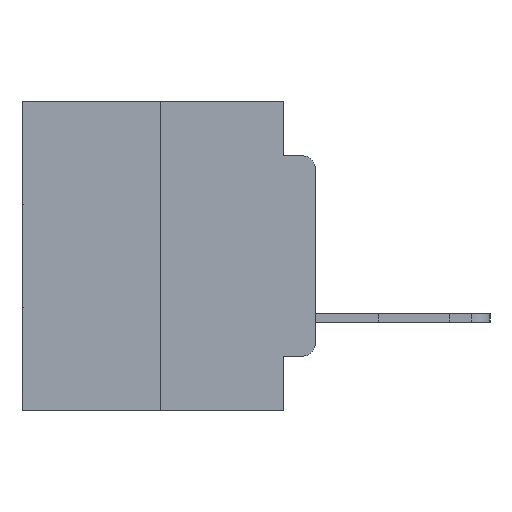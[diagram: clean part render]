
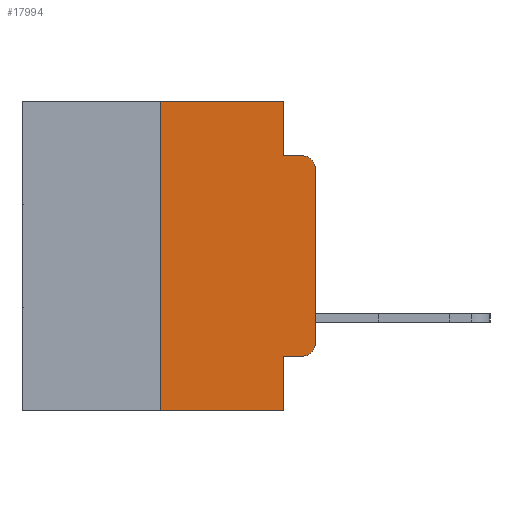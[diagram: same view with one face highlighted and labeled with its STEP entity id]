
A CAD part, left-side view. The second image highlights one B-rep face of the part: STEP entity #17994.
In plain terms, the highlighted planar face has unit normal (-1, 0, 0).
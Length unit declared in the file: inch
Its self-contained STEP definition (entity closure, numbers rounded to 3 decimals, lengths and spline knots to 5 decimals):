
#185 = CARTESIAN_POINT ( 'NONE',  ( 0., 0.473, 0. ) ) ;
#382 = DIRECTION ( 'NONE',  ( 0., 0., -1. ) ) ;
#536 = EDGE_CURVE ( 'NONE', #22121, #20713, #11908, .T. ) ;
#639 = ORIENTED_EDGE ( 'NONE', *, *, #2009, .T. ) ;
#859 = ORIENTED_EDGE ( 'NONE', *, *, #536, .F. ) ;
#1043 = VECTOR ( 'NONE', #7865, 39.37008 ) ;
#1145 = CARTESIAN_POINT ( 'NONE',  ( 0., 0.02, -0.0885 ) ) ;
#1493 = CARTESIAN_POINT ( 'NONE',  ( 0., 0.02, -0.1085 ) ) ;
#1731 = VERTEX_POINT ( 'NONE', #24052 ) ;
#2009 = EDGE_CURVE ( 'NONE', #20157, #20713, #19663, .T. ) ;
#2152 = DIRECTION ( 'NONE',  ( 0., 0., -1. ) ) ;
#2168 = ORIENTED_EDGE ( 'NONE', *, *, #26574, .F. ) ;
#2206 = DIRECTION ( 'NONE',  ( -1., 0., 0. ) ) ;
#2355 = VERTEX_POINT ( 'NONE', #19625 ) ;
#2718 = ORIENTED_EDGE ( 'NONE', *, *, #15513, .F. ) ;
#2742 = ORIENTED_EDGE ( 'NONE', *, *, #23814, .F. ) ;
#3033 = CARTESIAN_POINT ( 'NONE',  ( 0., 0.473, 0. ) ) ;
#3064 = ORIENTED_EDGE ( 'NONE', *, *, #19917, .T. ) ;
#3578 = ORIENTED_EDGE ( 'NONE', *, *, #22426, .F. ) ;
#3601 = ORIENTED_EDGE ( 'NONE', *, *, #18114, .T. ) ;
#4000 = ORIENTED_EDGE ( 'NONE', *, *, #16690, .T. ) ;
#4567 = ORIENTED_EDGE ( 'NONE', *, *, #4946, .T. ) ;
#4688 = FACE_OUTER_BOUND ( 'NONE', #20049, .T. ) ;
#4752 = VECTOR ( 'NONE', #19409, 39.37008 ) ;
#4816 = CARTESIAN_POINT ( 'NONE',  ( 0., 0.02, -0.3915 ) ) ;
#4850 = VECTOR ( 'NONE', #22303, 39.37008 ) ;
#4946 = EDGE_CURVE ( 'NONE', #26338, #20157, #15893, .T. ) ;
#5247 = DIRECTION ( 'NONE',  ( 1., 0., 0. ) ) ;
#5387 = LINE ( 'NONE', #23893, #21513 ) ;
#5728 = CARTESIAN_POINT ( 'NONE',  ( 0., 0.051, -0.4115 ) ) ;
#6226 = LINE ( 'NONE', #20135, #4850 ) ;
#6451 = AXIS2_PLACEMENT_3D ( 'NONE', #1493, #2206, #2152 ) ;
#6827 = LINE ( 'NONE', #5728, #1043 ) ;
#6956 = DIRECTION ( 'NONE',  ( 0., 0., -1. ) ) ;
#7335 = DIRECTION ( 'NONE',  ( 0., 0., -1. ) ) ;
#7837 = CARTESIAN_POINT ( 'NONE',  ( 0., 0., -0.1085 ) ) ;
#7865 = DIRECTION ( 'NONE',  ( 0., -1., 0. ) ) ;
#8996 = AXIS2_PLACEMENT_3D ( 'NONE', #4816, #19517, #6956 ) ;
#11908 = LINE ( 'NONE', #23464, #16736 ) ;
#12832 = VERTEX_POINT ( 'NONE', #24015 ) ;
#13023 = CARTESIAN_POINT ( 'NONE',  ( 0., 0., 0. ) ) ;
#13502 = CARTESIAN_POINT ( 'NONE',  ( 0., 0.25, -0.5 ) ) ;
#13549 = DIRECTION ( 'NONE',  ( 0., -1., 0. ) ) ;
#13653 = CARTESIAN_POINT ( 'NONE',  ( 0., 0.051, 0. ) ) ;
#13824 = VECTOR ( 'NONE', #7335, 39.37008 ) ;
#14417 = VERTEX_POINT ( 'NONE', #13502 ) ;
#15513 = EDGE_CURVE ( 'NONE', #19841, #2355, #19642, .T. ) ;
#15685 = PLANE ( 'NONE',  #18059 ) ;
#15893 = LINE ( 'NONE', #13023, #4752 ) ;
#16690 = EDGE_CURVE ( 'NONE', #1731, #26338, #26442, .T. ) ;
#16736 = VECTOR ( 'NONE', #13549, 39.37008 ) ;
#17994 = ADVANCED_FACE ( 'NONE', ( #4688 ), #15685, .F. ) ;
#18059 = AXIS2_PLACEMENT_3D ( 'NONE', #3033, #5247, #19937 ) ;
#18114 = EDGE_CURVE ( 'NONE', #19551, #1731, #6827, .T. ) ;
#18753 = VECTOR ( 'NONE', #382, 39.37008 ) ;
#19409 = DIRECTION ( 'NONE',  ( 0., 0., 1. ) ) ;
#19517 = DIRECTION ( 'NONE',  ( -1., 0., 0. ) ) ;
#19551 = VERTEX_POINT ( 'NONE', #21177 ) ;
#19625 = CARTESIAN_POINT ( 'NONE',  ( 0., 0.051, 0. ) ) ;
#19642 = LINE ( 'NONE', #185, #25867 ) ;
#19663 = CIRCLE ( 'NONE', #6451, 0.02 ) ;
#19841 = VERTEX_POINT ( 'NONE', #22290 ) ;
#19917 = EDGE_CURVE ( 'NONE', #14417, #12832, #5387, .T. ) ;
#19937 = DIRECTION ( 'NONE',  ( 0., 0., -1. ) ) ;
#20049 = EDGE_LOOP ( 'NONE', ( #4567, #639, #859, #2168, #2718, #2742, #3064, #3578, #3601, #4000 ) ) ;
#20135 = CARTESIAN_POINT ( 'NONE',  ( 0., 0.25, 0. ) ) ;
#20157 = VERTEX_POINT ( 'NONE', #7837 ) ;
#20713 = VERTEX_POINT ( 'NONE', #1145 ) ;
#21177 = CARTESIAN_POINT ( 'NONE',  ( 0., 0.051, -0.4115 ) ) ;
#21359 = DIRECTION ( 'NONE',  ( 0., -1., 0. ) ) ;
#21513 = VECTOR ( 'NONE', #25948, 39.37008 ) ;
#22121 = VERTEX_POINT ( 'NONE', #23064 ) ;
#22290 = CARTESIAN_POINT ( 'NONE',  ( 0., 0.25, 0. ) ) ;
#22303 = DIRECTION ( 'NONE',  ( 0., 0., 1. ) ) ;
#22426 = EDGE_CURVE ( 'NONE', #19551, #12832, #24985, .T. ) ;
#22774 = CARTESIAN_POINT ( 'NONE',  ( 0., 0., -0.3915 ) ) ;
#23064 = CARTESIAN_POINT ( 'NONE',  ( 0., 0.051, -0.0885 ) ) ;
#23464 = CARTESIAN_POINT ( 'NONE',  ( 0., 0.051, -0.0885 ) ) ;
#23814 = EDGE_CURVE ( 'NONE', #14417, #19841, #6226, .T. ) ;
#23893 = CARTESIAN_POINT ( 'NONE',  ( 0., 0.473, -0.5 ) ) ;
#24015 = CARTESIAN_POINT ( 'NONE',  ( 0., 0.051, -0.5 ) ) ;
#24052 = CARTESIAN_POINT ( 'NONE',  ( 0., 0.02, -0.4115 ) ) ;
#24985 = LINE ( 'NONE', #13653, #13824 ) ;
#25023 = LINE ( 'NONE', #25721, #18753 ) ;
#25721 = CARTESIAN_POINT ( 'NONE',  ( 0., 0.051, 0. ) ) ;
#25867 = VECTOR ( 'NONE', #21359, 39.37008 ) ;
#25948 = DIRECTION ( 'NONE',  ( 0., -1., 0. ) ) ;
#26338 = VERTEX_POINT ( 'NONE', #22774 ) ;
#26442 = CIRCLE ( 'NONE', #8996, 0.02 ) ;
#26574 = EDGE_CURVE ( 'NONE', #2355, #22121, #25023, .T. ) ;
